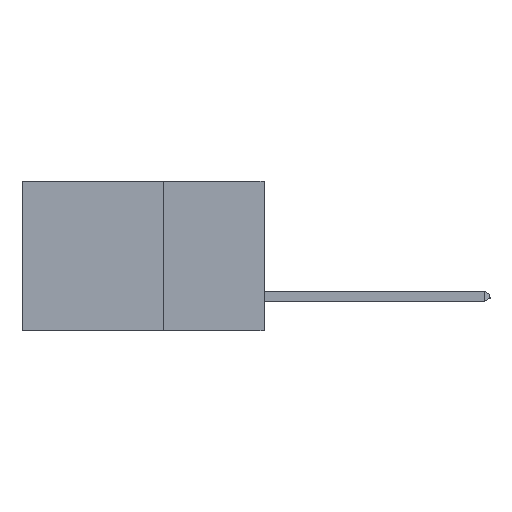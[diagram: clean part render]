
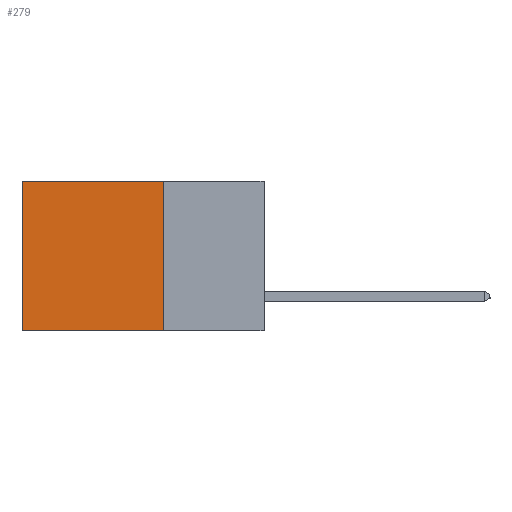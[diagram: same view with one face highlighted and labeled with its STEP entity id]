
A CAD part, left-side view. The second image highlights one B-rep face of the part: STEP entity #279.
In plain terms, the highlighted planar face has unit normal (-1, 0, 0).
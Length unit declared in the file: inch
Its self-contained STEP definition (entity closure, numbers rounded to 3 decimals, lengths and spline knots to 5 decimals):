
#279 = ADVANCED_FACE ( 'NONE', ( #22636 ), #13078, .F. ) ;
#469 = VERTEX_POINT ( 'NONE', #27233 ) ;
#1048 = CARTESIAN_POINT ( 'NONE',  ( 0.298, 0.25, 0. ) ) ;
#2092 = EDGE_CURVE ( 'NONE', #20820, #469, #26528, .T. ) ;
#4587 = DIRECTION ( 'NONE',  ( 0., 1., 0. ) ) ;
#5331 = DIRECTION ( 'NONE',  ( 1., 0., 0. ) ) ;
#5700 = LINE ( 'NONE', #20114, #18019 ) ;
#5953 = VERTEX_POINT ( 'NONE', #13227 ) ;
#6469 = ORIENTED_EDGE ( 'NONE', *, *, #25907, .F. ) ;
#8283 = DIRECTION ( 'NONE',  ( 0., 0., -1. ) ) ;
#9126 = LINE ( 'NONE', #16503, #14289 ) ;
#10036 = VECTOR ( 'NONE', #21145, 39.37008 ) ;
#10480 = LINE ( 'NONE', #23992, #20661 ) ;
#10856 = CARTESIAN_POINT ( 'NONE',  ( 0.298, 0.25, 0. ) ) ;
#13078 = PLANE ( 'NONE',  #17983 ) ;
#13227 = CARTESIAN_POINT ( 'NONE',  ( 0.298, 0.6, 0. ) ) ;
#13713 = ORIENTED_EDGE ( 'NONE', *, *, #15414, .T. ) ;
#14289 = VECTOR ( 'NONE', #18683, 39.37008 ) ;
#15414 = EDGE_CURVE ( 'NONE', #5953, #23632, #5700, .T. ) ;
#16503 = CARTESIAN_POINT ( 'NONE',  ( 0.298, 0.25, 0. ) ) ;
#16942 = EDGE_LOOP ( 'NONE', ( #13713, #6469, #25067, #22108 ) ) ;
#17983 = AXIS2_PLACEMENT_3D ( 'NONE', #1048, #5331, #8283 ) ;
#18019 = VECTOR ( 'NONE', #20027, 39.37008 ) ;
#18683 = DIRECTION ( 'NONE',  ( 0., 1., 0. ) ) ;
#20027 = DIRECTION ( 'NONE',  ( 0., 0., -1. ) ) ;
#20114 = CARTESIAN_POINT ( 'NONE',  ( 0.298, 0.6, 0. ) ) ;
#20661 = VECTOR ( 'NONE', #4587, 39.37008 ) ;
#20719 = CARTESIAN_POINT ( 'NONE',  ( 0.298, 0.25, 0. ) ) ;
#20820 = VERTEX_POINT ( 'NONE', #20719 ) ;
#21145 = DIRECTION ( 'NONE',  ( 0., 0., -1. ) ) ;
#22108 = ORIENTED_EDGE ( 'NONE', *, *, #25501, .T. ) ;
#22636 = FACE_OUTER_BOUND ( 'NONE', #16942, .T. ) ;
#23632 = VERTEX_POINT ( 'NONE', #27694 ) ;
#23992 = CARTESIAN_POINT ( 'NONE',  ( 0.298, 0.25, -0.37 ) ) ;
#25067 = ORIENTED_EDGE ( 'NONE', *, *, #2092, .F. ) ;
#25501 = EDGE_CURVE ( 'NONE', #20820, #5953, #9126, .T. ) ;
#25907 = EDGE_CURVE ( 'NONE', #469, #23632, #10480, .T. ) ;
#26528 = LINE ( 'NONE', #10856, #10036 ) ;
#27233 = CARTESIAN_POINT ( 'NONE',  ( 0.298, 0.25, -0.37 ) ) ;
#27694 = CARTESIAN_POINT ( 'NONE',  ( 0.298, 0.6, -0.37 ) ) ;
